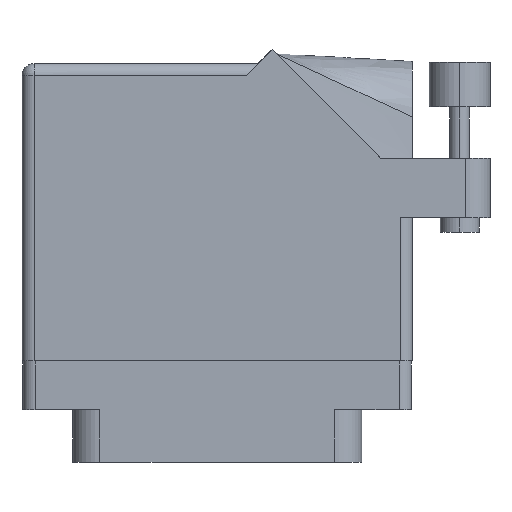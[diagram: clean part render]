
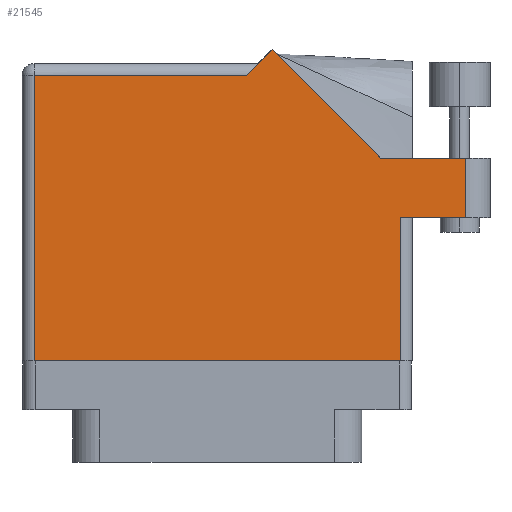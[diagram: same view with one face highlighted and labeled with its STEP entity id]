
A CAD part, front view. The second image highlights one B-rep face of the part: STEP entity #21545.
In plain terms, the highlighted face is planar.
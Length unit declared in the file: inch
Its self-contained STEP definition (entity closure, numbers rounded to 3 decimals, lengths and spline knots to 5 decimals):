
#430 = PLANE ( 'NONE',  #9545 ) ;
#668 = CARTESIAN_POINT ( 'NONE',  ( -1.005, 1.43, 0.455 ) ) ;
#669 = CARTESIAN_POINT ( 'NONE',  ( 0.15, 1.368, 0.455 ) ) ;
#945 = DIRECTION ( 'NONE',  ( -1., 0., 0. ) ) ;
#1026 = CARTESIAN_POINT ( 'NONE',  ( 0.83942, 0.944, 0.455 ) ) ;
#1484 = EDGE_CURVE ( 'NONE', #3454, #32147, #21131, .T. ) ;
#1637 = ORIENTED_EDGE ( 'NONE', *, *, #7018, .T. ) ;
#2720 = ORIENTED_EDGE ( 'NONE', *, *, #10725, .T. ) ;
#3203 = CARTESIAN_POINT ( 'NONE',  ( 1.28, 0.944, 0.455 ) ) ;
#3229 = VERTEX_POINT ( 'NONE', #29343 ) ;
#3454 = VERTEX_POINT ( 'NONE', #20790 ) ;
#3493 = CARTESIAN_POINT ( 'NONE',  ( 1.405, 0.944, 0.455 ) ) ;
#3611 = ORIENTED_EDGE ( 'NONE', *, *, #1484, .T. ) ;
#3766 = LINE ( 'NONE', #26342, #5129 ) ;
#4050 = DIRECTION ( 'NONE',  ( 1., 0., 0. ) ) ;
#4102 = CARTESIAN_POINT ( 'NONE',  ( 0.943, 0.637, 0.455 ) ) ;
#4264 = ORIENTED_EDGE ( 'NONE', *, *, #26276, .T. ) ;
#5129 = VECTOR ( 'NONE', #18081, 39.37008 ) ;
#5502 = ORIENTED_EDGE ( 'NONE', *, *, #24645, .T. ) ;
#6056 = ORIENTED_EDGE ( 'NONE', *, *, #28603, .T. ) ;
#6377 = VERTEX_POINT ( 'NONE', #17272 ) ;
#7018 = EDGE_CURVE ( 'NONE', #11078, #3229, #3766, .T. ) ;
#7064 = ORIENTED_EDGE ( 'NONE', *, *, #20983, .T. ) ;
#7102 = DIRECTION ( 'NONE',  ( 0., 1., 0. ) ) ;
#8361 = VECTOR ( 'NONE', #15136, 39.37008 ) ;
#8984 = FACE_OUTER_BOUND ( 'NONE', #28548, .T. ) ;
#9465 = CARTESIAN_POINT ( 'NONE',  ( -1.005, -0.1, 0.455 ) ) ;
#9508 = DIRECTION ( 'NONE',  ( 0., -1., 0. ) ) ;
#9545 = AXIS2_PLACEMENT_3D ( 'NONE', #668, #14256, #33718 ) ;
#10725 = EDGE_CURVE ( 'NONE', #6377, #3454, #17287, .T. ) ;
#11047 = VERTEX_POINT ( 'NONE', #14257 ) ;
#11078 = VERTEX_POINT ( 'NONE', #669 ) ;
#11203 = EDGE_CURVE ( 'NONE', #34480, #6377, #16788, .T. ) ;
#12206 = DIRECTION ( 'NONE',  ( -0.707, -0.707, 0. ) ) ;
#12325 = CARTESIAN_POINT ( 'NONE',  ( 1.28, 0.944, 0.455 ) ) ;
#14256 = DIRECTION ( 'NONE',  ( 0., 0., -1. ) ) ;
#14257 = CARTESIAN_POINT ( 'NONE',  ( 0.28271, 1.50071, 0.455 ) ) ;
#15136 = DIRECTION ( 'NONE',  ( -0.707, 0.707, 0. ) ) ;
#16788 = LINE ( 'NONE', #9465, #34606 ) ;
#17272 = CARTESIAN_POINT ( 'NONE',  ( 0.943, -0.1, 0.455 ) ) ;
#17287 = LINE ( 'NONE', #4102, #21226 ) ;
#17918 = CARTESIAN_POINT ( 'NONE',  ( 1.005, 0.637, 0.455 ) ) ;
#17949 = CARTESIAN_POINT ( 'NONE',  ( 0.83942, 0.944, 0.455 ) ) ;
#18081 = DIRECTION ( 'NONE',  ( -1., 0., 0. ) ) ;
#19704 = VECTOR ( 'NONE', #7102, 39.37008 ) ;
#20292 = CARTESIAN_POINT ( 'NONE',  ( -0.943, -0.1, 0.455 ) ) ;
#20790 = CARTESIAN_POINT ( 'NONE',  ( 0.943, 0.637, 0.455 ) ) ;
#20983 = EDGE_CURVE ( 'NONE', #3229, #34480, #32993, .T. ) ;
#21131 = LINE ( 'NONE', #17918, #35025 ) ;
#21226 = VECTOR ( 'NONE', #29378, 39.37008 ) ;
#21545 = ADVANCED_FACE ( 'NONE', ( #8984 ), #430, .F. ) ;
#21929 = CARTESIAN_POINT ( 'NONE',  ( -0.943, -0.1, 0.455 ) ) ;
#22321 = LINE ( 'NONE', #17949, #8361 ) ;
#23289 = DIRECTION ( 'NONE',  ( 1., 0., 0. ) ) ;
#24362 = EDGE_CURVE ( 'NONE', #30358, #11047, #22321, .T. ) ;
#24451 = ORIENTED_EDGE ( 'NONE', *, *, #24362, .T. ) ;
#24645 = EDGE_CURVE ( 'NONE', #32147, #35779, #30959, .T. ) ;
#24718 = ORIENTED_EDGE ( 'NONE', *, *, #11203, .T. ) ;
#26212 = CARTESIAN_POINT ( 'NONE',  ( 0.212, 1.43, 0.455 ) ) ;
#26276 = EDGE_CURVE ( 'NONE', #11047, #11078, #28135, .T. ) ;
#26342 = CARTESIAN_POINT ( 'NONE',  ( -1.005, 1.368, 0.455 ) ) ;
#28135 = LINE ( 'NONE', #26212, #32035 ) ;
#28548 = EDGE_LOOP ( 'NONE', ( #3611, #5502, #6056, #24451, #4264, #1637, #7064, #24718, #2720 ) ) ;
#28603 = EDGE_CURVE ( 'NONE', #35779, #30358, #30976, .T. ) ;
#28667 = VECTOR ( 'NONE', #9508, 39.37008 ) ;
#29343 = CARTESIAN_POINT ( 'NONE',  ( -0.943, 1.368, 0.455 ) ) ;
#29378 = DIRECTION ( 'NONE',  ( 0., 1., 0. ) ) ;
#30358 = VERTEX_POINT ( 'NONE', #1026 ) ;
#30508 = CARTESIAN_POINT ( 'NONE',  ( 1.28, 0.637, 0.455 ) ) ;
#30959 = LINE ( 'NONE', #12325, #19704 ) ;
#30976 = LINE ( 'NONE', #3493, #33157 ) ;
#32035 = VECTOR ( 'NONE', #12206, 39.37008 ) ;
#32147 = VERTEX_POINT ( 'NONE', #30508 ) ;
#32993 = LINE ( 'NONE', #20292, #28667 ) ;
#33157 = VECTOR ( 'NONE', #945, 39.37008 ) ;
#33718 = DIRECTION ( 'NONE',  ( -1., 0., 0. ) ) ;
#34480 = VERTEX_POINT ( 'NONE', #21929 ) ;
#34606 = VECTOR ( 'NONE', #4050, 39.37008 ) ;
#35025 = VECTOR ( 'NONE', #23289, 39.37008 ) ;
#35779 = VERTEX_POINT ( 'NONE', #3203 ) ;
